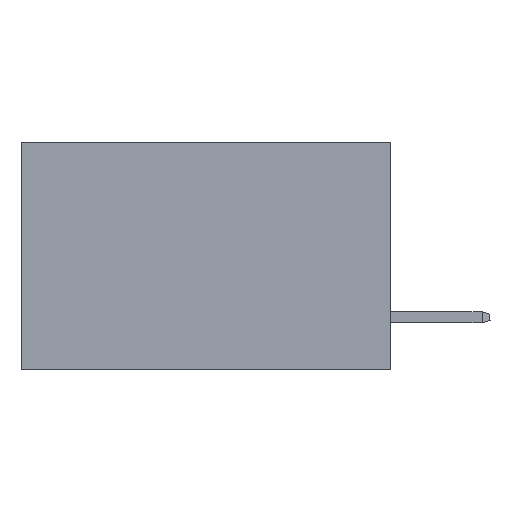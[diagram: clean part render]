
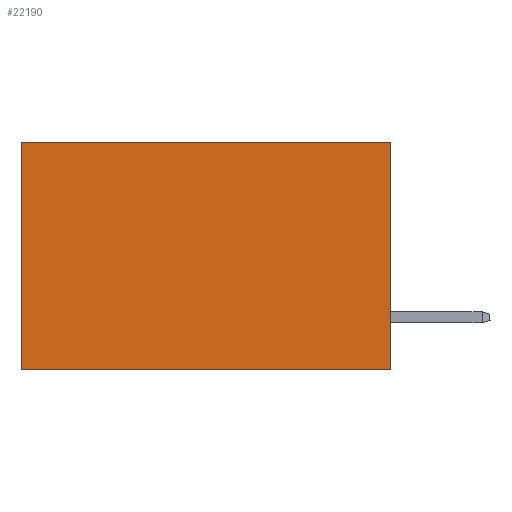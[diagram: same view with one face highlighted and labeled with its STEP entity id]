
A CAD part, left-side view. The second image highlights one B-rep face of the part: STEP entity #22190.
In plain terms, the highlighted planar face has unit normal (-1, 0, 0).
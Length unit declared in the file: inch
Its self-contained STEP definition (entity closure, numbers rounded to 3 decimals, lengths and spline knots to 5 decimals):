
#140 = EDGE_LOOP ( 'NONE', ( #15268, #2048, #14915, #24473 ) ) ;
#1210 = DIRECTION ( 'NONE',  ( 0., 1., 0. ) ) ;
#2048 = ORIENTED_EDGE ( 'NONE', *, *, #22783, .F. ) ;
#2545 = VECTOR ( 'NONE', #20322, 39.37008 ) ;
#3507 = CARTESIAN_POINT ( 'NONE',  ( 0.2875, 0.6, 0. ) ) ;
#5139 = VECTOR ( 'NONE', #7574, 39.37008 ) ;
#5784 = VECTOR ( 'NONE', #1210, 39.37008 ) ;
#6014 = VERTEX_POINT ( 'NONE', #24683 ) ;
#7574 = DIRECTION ( 'NONE',  ( 0., 0., -1. ) ) ;
#7853 = LINE ( 'NONE', #24416, #2545 ) ;
#8812 = FACE_OUTER_BOUND ( 'NONE', #140, .T. ) ;
#8855 = LINE ( 'NONE', #3507, #5139 ) ;
#10063 = VERTEX_POINT ( 'NONE', #18072 ) ;
#10436 = DIRECTION ( 'NONE',  ( 0., 0., -1. ) ) ;
#11221 = AXIS2_PLACEMENT_3D ( 'NONE', #25707, #22011, #13833 ) ;
#11446 = LINE ( 'NONE', #17139, #5784 ) ;
#12039 = CARTESIAN_POINT ( 'NONE',  ( 0.2875, 0.6, -0.37 ) ) ;
#13833 = DIRECTION ( 'NONE',  ( 0., 0., -1. ) ) ;
#14062 = EDGE_CURVE ( 'NONE', #10063, #25549, #16513, .T. ) ;
#14278 = VERTEX_POINT ( 'NONE', #12039 ) ;
#14915 = ORIENTED_EDGE ( 'NONE', *, *, #14062, .F. ) ;
#15268 = ORIENTED_EDGE ( 'NONE', *, *, #21320, .T. ) ;
#16196 = EDGE_CURVE ( 'NONE', #10063, #6014, #11446, .T. ) ;
#16513 = LINE ( 'NONE', #18386, #23671 ) ;
#16767 = CARTESIAN_POINT ( 'NONE',  ( 0.2875, 0., -0.37 ) ) ;
#17139 = CARTESIAN_POINT ( 'NONE',  ( 0.2875, 0., 0. ) ) ;
#18072 = CARTESIAN_POINT ( 'NONE',  ( 0.2875, 0., 0. ) ) ;
#18386 = CARTESIAN_POINT ( 'NONE',  ( 0.2875, 0., 0. ) ) ;
#20322 = DIRECTION ( 'NONE',  ( 0., 1., 0. ) ) ;
#21320 = EDGE_CURVE ( 'NONE', #6014, #14278, #8855, .T. ) ;
#22011 = DIRECTION ( 'NONE',  ( 1., 0., 0. ) ) ;
#22190 = ADVANCED_FACE ( 'NONE', ( #8812 ), #23704, .F. ) ;
#22783 = EDGE_CURVE ( 'NONE', #25549, #14278, #7853, .T. ) ;
#23671 = VECTOR ( 'NONE', #10436, 39.37008 ) ;
#23704 = PLANE ( 'NONE',  #11221 ) ;
#24416 = CARTESIAN_POINT ( 'NONE',  ( 0.2875, 0., -0.37 ) ) ;
#24473 = ORIENTED_EDGE ( 'NONE', *, *, #16196, .T. ) ;
#24683 = CARTESIAN_POINT ( 'NONE',  ( 0.2875, 0.6, 0. ) ) ;
#25549 = VERTEX_POINT ( 'NONE', #16767 ) ;
#25707 = CARTESIAN_POINT ( 'NONE',  ( 0.2875, 0., 0. ) ) ;
